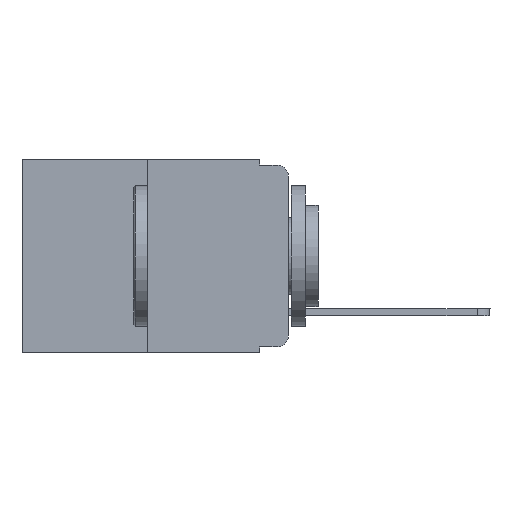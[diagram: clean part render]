
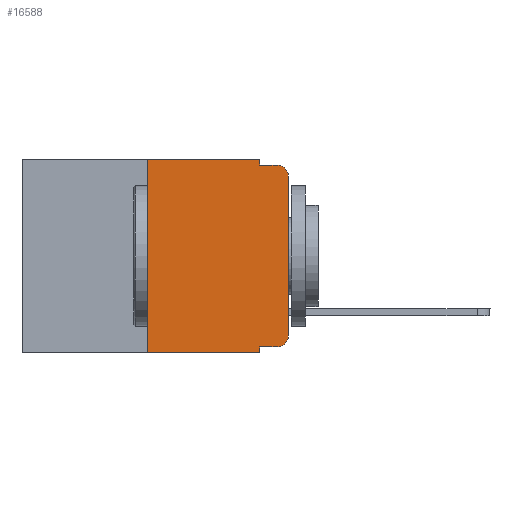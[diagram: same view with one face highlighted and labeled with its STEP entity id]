
A CAD part, left-side view. The second image highlights one B-rep face of the part: STEP entity #16588.
In plain terms, the highlighted planar face has unit normal (-1, 0, 0).
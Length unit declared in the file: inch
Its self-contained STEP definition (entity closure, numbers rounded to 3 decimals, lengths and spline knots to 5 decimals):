
#19 = LINE ( 'NONE', #1323, #5112 ) ;
#186 = VERTEX_POINT ( 'NONE', #14903 ) ;
#628 = CARTESIAN_POINT ( 'NONE',  ( 0., 0.051, 0. ) ) ;
#1071 = CARTESIAN_POINT ( 'NONE',  ( 0., 0.02, -0.03 ) ) ;
#1227 = CARTESIAN_POINT ( 'NONE',  ( 0., 0.051, 0. ) ) ;
#1323 = CARTESIAN_POINT ( 'NONE',  ( 0., 0.473, 0. ) ) ;
#1468 = LINE ( 'NONE', #9489, #4804 ) ;
#1706 = CARTESIAN_POINT ( 'NONE',  ( 0., 0.25, 0. ) ) ;
#1707 = VERTEX_POINT ( 'NONE', #4325 ) ;
#1973 = CARTESIAN_POINT ( 'NONE',  ( 0., 0.473, 0. ) ) ;
#2022 = DIRECTION ( 'NONE',  ( 0., 0., -1. ) ) ;
#2072 = VERTEX_POINT ( 'NONE', #14525 ) ;
#2239 = DIRECTION ( 'NONE',  ( 0., -1., 0. ) ) ;
#2645 = VERTEX_POINT ( 'NONE', #15115 ) ;
#2865 = EDGE_LOOP ( 'NONE', ( #16156, #6747, #3375, #5533, #9953, #11055, #16580, #3583, #12910, #9915 ) ) ;
#3042 = AXIS2_PLACEMENT_3D ( 'NONE', #1071, #11697, #14311 ) ;
#3304 = VERTEX_POINT ( 'NONE', #5493 ) ;
#3375 = ORIENTED_EDGE ( 'NONE', *, *, #16329, .F. ) ;
#3583 = ORIENTED_EDGE ( 'NONE', *, *, #13703, .F. ) ;
#4325 = CARTESIAN_POINT ( 'NONE',  ( 0., 0.25, -0.343 ) ) ;
#4336 = FACE_OUTER_BOUND ( 'NONE', #2865, .T. ) ;
#4489 = DIRECTION ( 'NONE',  ( 0., 0., 1. ) ) ;
#4657 = DIRECTION ( 'NONE',  ( 0., 0., -1. ) ) ;
#4804 = VECTOR ( 'NONE', #11999, 39.37008 ) ;
#5112 = VECTOR ( 'NONE', #10479, 39.37008 ) ;
#5204 = VECTOR ( 'NONE', #6763, 39.37008 ) ;
#5493 = CARTESIAN_POINT ( 'NONE',  ( 0., 0.25, 0. ) ) ;
#5533 = ORIENTED_EDGE ( 'NONE', *, *, #10256, .F. ) ;
#5839 = CIRCLE ( 'NONE', #10020, 0.02 ) ;
#5882 = LINE ( 'NONE', #1706, #10771 ) ;
#5928 = CARTESIAN_POINT ( 'NONE',  ( 0., 0.051, -0.343 ) ) ;
#6283 = DIRECTION ( 'NONE',  ( 0., 0., -1. ) ) ;
#6747 = ORIENTED_EDGE ( 'NONE', *, *, #7132, .T. ) ;
#6763 = DIRECTION ( 'NONE',  ( 0., 0., 1. ) ) ;
#6949 = DIRECTION ( 'NONE',  ( 0., 0., -1. ) ) ;
#7132 = EDGE_CURVE ( 'NONE', #2072, #7154, #7220, .T. ) ;
#7154 = VERTEX_POINT ( 'NONE', #12904 ) ;
#7220 = CIRCLE ( 'NONE', #3042, 0.02 ) ;
#8084 = EDGE_CURVE ( 'NONE', #8184, #2645, #10437, .T. ) ;
#8086 = VECTOR ( 'NONE', #2239, 39.37008 ) ;
#8184 = VERTEX_POINT ( 'NONE', #8304 ) ;
#8304 = CARTESIAN_POINT ( 'NONE',  ( 0., 0.051, -0.333 ) ) ;
#8823 = CARTESIAN_POINT ( 'NONE',  ( 0., 0.051, 0. ) ) ;
#8918 = EDGE_CURVE ( 'NONE', #2645, #186, #5839, .T. ) ;
#9212 = LINE ( 'NONE', #13452, #5204 ) ;
#9283 = VECTOR ( 'NONE', #2022, 39.37008 ) ;
#9489 = CARTESIAN_POINT ( 'NONE',  ( 0., 0.473, -0.343 ) ) ;
#9915 = ORIENTED_EDGE ( 'NONE', *, *, #8918, .T. ) ;
#9953 = ORIENTED_EDGE ( 'NONE', *, *, #12510, .F. ) ;
#10020 = AXIS2_PLACEMENT_3D ( 'NONE', #12806, #10293, #6283 ) ;
#10256 = EDGE_CURVE ( 'NONE', #12379, #14320, #11681, .T. ) ;
#10267 = CARTESIAN_POINT ( 'NONE',  ( 0., 0.051, -0.333 ) ) ;
#10293 = DIRECTION ( 'NONE',  ( -1., 0., 0. ) ) ;
#10313 = LINE ( 'NONE', #8823, #9283 ) ;
#10370 = CARTESIAN_POINT ( 'NONE',  ( 0., 0.051, -0.01 ) ) ;
#10437 = LINE ( 'NONE', #10267, #8086 ) ;
#10479 = DIRECTION ( 'NONE',  ( 0., -1., 0. ) ) ;
#10771 = VECTOR ( 'NONE', #4489, 39.37008 ) ;
#11055 = ORIENTED_EDGE ( 'NONE', *, *, #17064, .F. ) ;
#11182 = EDGE_CURVE ( 'NONE', #1707, #14006, #1468, .T. ) ;
#11444 = VECTOR ( 'NONE', #4657, 39.37008 ) ;
#11681 = LINE ( 'NONE', #1227, #11444 ) ;
#11697 = DIRECTION ( 'NONE',  ( -1., 0., 0. ) ) ;
#11999 = DIRECTION ( 'NONE',  ( 0., -1., 0. ) ) ;
#12263 = CARTESIAN_POINT ( 'NONE',  ( 0., 0.051, -0.01 ) ) ;
#12379 = VERTEX_POINT ( 'NONE', #628 ) ;
#12510 = EDGE_CURVE ( 'NONE', #3304, #12379, #19, .T. ) ;
#12600 = DIRECTION ( 'NONE',  ( 1., 0., 0. ) ) ;
#12806 = CARTESIAN_POINT ( 'NONE',  ( 0., 0.02, -0.313 ) ) ;
#12904 = CARTESIAN_POINT ( 'NONE',  ( 0., 0.02, -0.01 ) ) ;
#12910 = ORIENTED_EDGE ( 'NONE', *, *, #8084, .T. ) ;
#13452 = CARTESIAN_POINT ( 'NONE',  ( 0., 0., 0. ) ) ;
#13703 = EDGE_CURVE ( 'NONE', #8184, #14006, #10313, .T. ) ;
#14006 = VERTEX_POINT ( 'NONE', #5928 ) ;
#14311 = DIRECTION ( 'NONE',  ( 0., 0., -1. ) ) ;
#14320 = VERTEX_POINT ( 'NONE', #12263 ) ;
#14525 = CARTESIAN_POINT ( 'NONE',  ( 0., 0., -0.03 ) ) ;
#14903 = CARTESIAN_POINT ( 'NONE',  ( 0., 0., -0.313 ) ) ;
#15115 = CARTESIAN_POINT ( 'NONE',  ( 0., 0.02, -0.333 ) ) ;
#15705 = DIRECTION ( 'NONE',  ( 0., -1., 0. ) ) ;
#16066 = VECTOR ( 'NONE', #15705, 39.37008 ) ;
#16156 = ORIENTED_EDGE ( 'NONE', *, *, #16920, .T. ) ;
#16276 = PLANE ( 'NONE',  #16315 ) ;
#16315 = AXIS2_PLACEMENT_3D ( 'NONE', #1973, #12600, #6949 ) ;
#16329 = EDGE_CURVE ( 'NONE', #14320, #7154, #17000, .T. ) ;
#16580 = ORIENTED_EDGE ( 'NONE', *, *, #11182, .T. ) ;
#16588 = ADVANCED_FACE ( 'NONE', ( #4336 ), #16276, .F. ) ;
#16920 = EDGE_CURVE ( 'NONE', #186, #2072, #9212, .T. ) ;
#17000 = LINE ( 'NONE', #10370, #16066 ) ;
#17064 = EDGE_CURVE ( 'NONE', #1707, #3304, #5882, .T. ) ;
